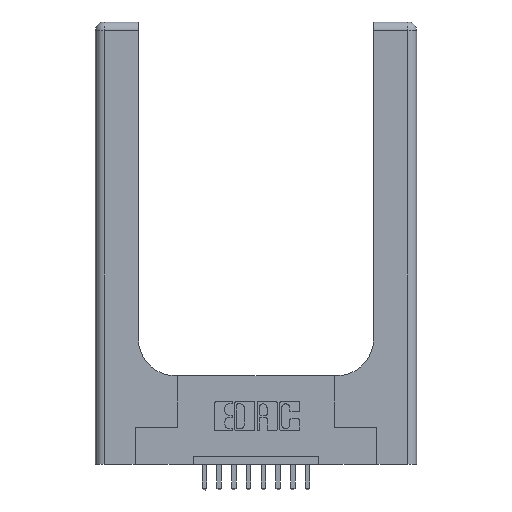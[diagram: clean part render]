
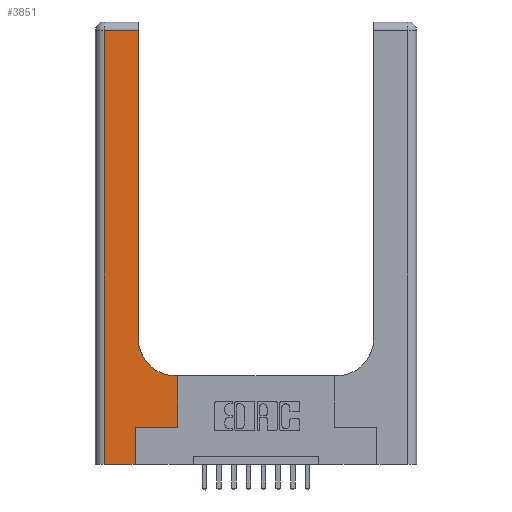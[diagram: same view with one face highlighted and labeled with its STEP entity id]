
A CAD part, top view. The second image highlights one B-rep face of the part: STEP entity #3851.
In plain terms, the highlighted planar face has unit normal (0, 0, 1).
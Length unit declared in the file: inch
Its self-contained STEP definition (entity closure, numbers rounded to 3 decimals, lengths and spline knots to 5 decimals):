
#41 = CARTESIAN_POINT ( 'NONE',  ( 0.2915, 0.85, 0.37 ) ) ;
#60 = VERTEX_POINT ( 'NONE', #9180 ) ;
#123 = CARTESIAN_POINT ( 'NONE',  ( 0.5415, 0.85, 0.37 ) ) ;
#125 = ORIENTED_EDGE ( 'NONE', *, *, #1026, .T. ) ;
#471 = CARTESIAN_POINT ( 'NONE',  ( 0.2915, 0.6, 0.37 ) ) ;
#516 = EDGE_CURVE ( 'NONE', #1299, #5281, #3487, .T. ) ;
#575 = DIRECTION ( 'NONE',  ( 0., 1., 0. ) ) ;
#642 = VERTEX_POINT ( 'NONE', #5414 ) ;
#657 = CARTESIAN_POINT ( 'NONE',  ( 0.269, 0., 0.37 ) ) ;
#750 = LINE ( 'NONE', #657, #15729 ) ;
#949 = EDGE_LOOP ( 'NONE', ( #125, #8603, #6302, #12778, #8647, #6203, #3109, #5824, #11846 ) ) ;
#1026 = EDGE_CURVE ( 'NONE', #15379, #1299, #6139, .T. ) ;
#1226 = CARTESIAN_POINT ( 'NONE',  ( 0.5585, 0.25, 0.37 ) ) ;
#1266 = LINE ( 'NONE', #471, #4928 ) ;
#1299 = VERTEX_POINT ( 'NONE', #11033 ) ;
#1309 = CIRCLE ( 'NONE', #9110, 0.25 ) ;
#1469 = DIRECTION ( 'NONE',  ( -1., 0., 0. ) ) ;
#1616 = EDGE_CURVE ( 'NONE', #2872, #1891, #15387, .T. ) ;
#1891 = VERTEX_POINT ( 'NONE', #9429 ) ;
#2157 = EDGE_CURVE ( 'NONE', #5540, #15379, #1309, .T. ) ;
#2233 = LINE ( 'NONE', #11161, #7422 ) ;
#2398 = DIRECTION ( 'NONE',  ( 1., 0., 0. ) ) ;
#2411 = DIRECTION ( 'NONE',  ( 0., 1., 0. ) ) ;
#2872 = VERTEX_POINT ( 'NONE', #15366 ) ;
#3109 = ORIENTED_EDGE ( 'NONE', *, *, #12919, .T. ) ;
#3243 = LINE ( 'NONE', #1226, #12712 ) ;
#3360 = AXIS2_PLACEMENT_3D ( 'NONE', #7107, #9670, #3455 ) ;
#3455 = DIRECTION ( 'NONE',  ( -1., 0., 0. ) ) ;
#3487 = LINE ( 'NONE', #11506, #4820 ) ;
#3770 = DIRECTION ( 'NONE',  ( 0., -1., 0. ) ) ;
#3851 = ADVANCED_FACE ( 'NONE', ( #14204 ), #14454, .F. ) ;
#4147 = EDGE_CURVE ( 'NONE', #5281, #60, #2233, .T. ) ;
#4671 = DIRECTION ( 'NONE',  ( 1., 0., 0. ) ) ;
#4702 = CARTESIAN_POINT ( 'NONE',  ( 0.269, 0.25, 0.37 ) ) ;
#4820 = VECTOR ( 'NONE', #1469, 39.37008 ) ;
#4928 = VECTOR ( 'NONE', #10309, 39.37008 ) ;
#5281 = VERTEX_POINT ( 'NONE', #8262 ) ;
#5317 = CARTESIAN_POINT ( 'NONE',  ( 0.269, 0., 0.37 ) ) ;
#5414 = CARTESIAN_POINT ( 'NONE',  ( 0.5585, 0.6, 0.37 ) ) ;
#5540 = VERTEX_POINT ( 'NONE', #15075 ) ;
#5639 = CARTESIAN_POINT ( 'NONE',  ( 0.2915, 3., 0.37 ) ) ;
#5824 = ORIENTED_EDGE ( 'NONE', *, *, #13898, .T. ) ;
#6139 = LINE ( 'NONE', #5639, #12942 ) ;
#6203 = ORIENTED_EDGE ( 'NONE', *, *, #1616, .T. ) ;
#6302 = ORIENTED_EDGE ( 'NONE', *, *, #4147, .T. ) ;
#6856 = EDGE_CURVE ( 'NONE', #60, #8932, #14455, .T. ) ;
#7107 = CARTESIAN_POINT ( 'NONE',  ( 0., 3., 0.37 ) ) ;
#7422 = VECTOR ( 'NONE', #3770, 39.37008 ) ;
#8262 = CARTESIAN_POINT ( 'NONE',  ( 0.06, 2.94, 0.37 ) ) ;
#8603 = ORIENTED_EDGE ( 'NONE', *, *, #516, .T. ) ;
#8647 = ORIENTED_EDGE ( 'NONE', *, *, #13321, .T. ) ;
#8932 = VERTEX_POINT ( 'NONE', #5317 ) ;
#9110 = AXIS2_PLACEMENT_3D ( 'NONE', #123, #13600, #2398 ) ;
#9180 = CARTESIAN_POINT ( 'NONE',  ( 0.06, 0., 0.37 ) ) ;
#9239 = DIRECTION ( 'NONE',  ( 0., 1., 0. ) ) ;
#9429 = CARTESIAN_POINT ( 'NONE',  ( 0.5585, 0.25, 0.37 ) ) ;
#9670 = DIRECTION ( 'NONE',  ( 0., 0., -1. ) ) ;
#10309 = DIRECTION ( 'NONE',  ( -1., 0., 0. ) ) ;
#10415 = VECTOR ( 'NONE', #4671, 39.37008 ) ;
#11033 = CARTESIAN_POINT ( 'NONE',  ( 0.2915, 2.94, 0.37 ) ) ;
#11161 = CARTESIAN_POINT ( 'NONE',  ( 0.06, 3., 0.37 ) ) ;
#11506 = CARTESIAN_POINT ( 'NONE',  ( 0., 2.94, 0.37 ) ) ;
#11846 = ORIENTED_EDGE ( 'NONE', *, *, #2157, .T. ) ;
#12024 = CARTESIAN_POINT ( 'NONE',  ( 0., 0., 0.37 ) ) ;
#12136 = VECTOR ( 'NONE', #15717, 39.37008 ) ;
#12712 = VECTOR ( 'NONE', #2411, 39.37008 ) ;
#12778 = ORIENTED_EDGE ( 'NONE', *, *, #6856, .T. ) ;
#12919 = EDGE_CURVE ( 'NONE', #1891, #642, #3243, .T. ) ;
#12942 = VECTOR ( 'NONE', #575, 39.37008 ) ;
#13321 = EDGE_CURVE ( 'NONE', #8932, #2872, #750, .T. ) ;
#13600 = DIRECTION ( 'NONE',  ( 0., 0., -1. ) ) ;
#13898 = EDGE_CURVE ( 'NONE', #642, #5540, #1266, .T. ) ;
#14204 = FACE_OUTER_BOUND ( 'NONE', #949, .T. ) ;
#14454 = PLANE ( 'NONE',  #3360 ) ;
#14455 = LINE ( 'NONE', #12024, #10415 ) ;
#15075 = CARTESIAN_POINT ( 'NONE',  ( 0.5415, 0.6, 0.37 ) ) ;
#15366 = CARTESIAN_POINT ( 'NONE',  ( 0.269, 0.25, 0.37 ) ) ;
#15379 = VERTEX_POINT ( 'NONE', #41 ) ;
#15387 = LINE ( 'NONE', #4702, #12136 ) ;
#15717 = DIRECTION ( 'NONE',  ( 1., 0., 0. ) ) ;
#15729 = VECTOR ( 'NONE', #9239, 39.37008 ) ;
